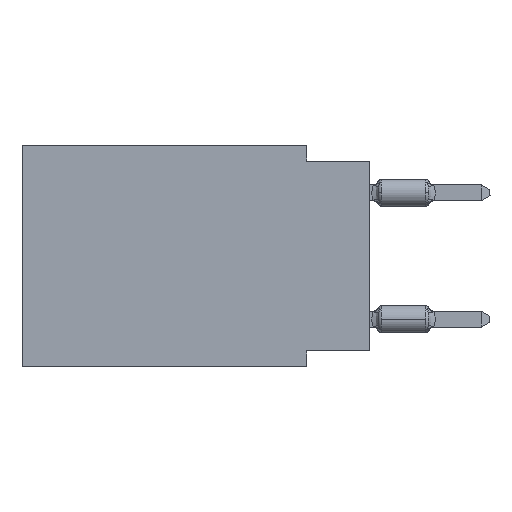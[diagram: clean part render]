
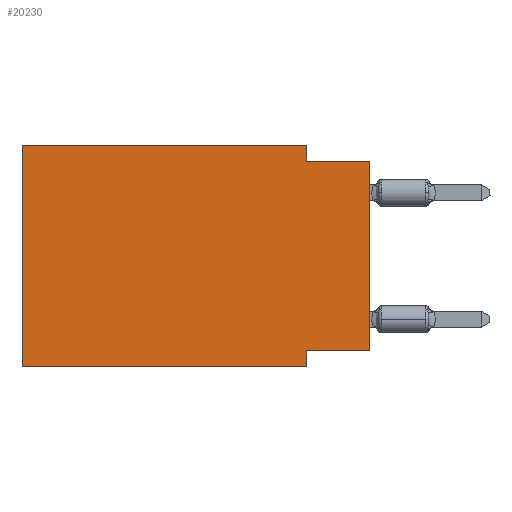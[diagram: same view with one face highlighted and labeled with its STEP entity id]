
A CAD part, left-side view. The second image highlights one B-rep face of the part: STEP entity #20230.
In plain terms, the highlighted planar face has unit normal (-1, 0, 0).
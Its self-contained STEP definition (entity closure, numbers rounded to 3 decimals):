
#2097 = ORIENTED_EDGE ( 'NONE', *, *, #26305, .F. ) ;
#3138 = DIRECTION ( 'NONE',  ( 0., 0., -1. ) ) ;
#5677 = DIRECTION ( 'NONE',  ( 0., 0., 1. ) ) ;
#6552 = VECTOR ( 'NONE', #24361, 1000. ) ;
#7790 = VERTEX_POINT ( 'NONE', #34208 ) ;
#7819 = VERTEX_POINT ( 'NONE', #51799 ) ;
#8036 = DIRECTION ( 'NONE',  ( 0., 0., 1. ) ) ;
#8139 = PLANE ( 'NONE',  #22504 ) ;
#8449 = EDGE_CURVE ( 'NONE', #12016, #8752, #50007, .T. ) ;
#8752 = VERTEX_POINT ( 'NONE', #41822 ) ;
#9020 = CARTESIAN_POINT ( 'NONE',  ( 0., 0., -8.255 ) ) ;
#9498 = VECTOR ( 'NONE', #8036, 1000. ) ;
#11505 = DIRECTION ( 'NONE',  ( 1., 0., 0. ) ) ;
#11742 = DIRECTION ( 'NONE',  ( 0., -1., 0. ) ) ;
#11849 = DIRECTION ( 'NONE',  ( 0., 0., -1. ) ) ;
#12016 = VERTEX_POINT ( 'NONE', #45140 ) ;
#12911 = ORIENTED_EDGE ( 'NONE', *, *, #34334, .F. ) ;
#14203 = LINE ( 'NONE', #52180, #38190 ) ;
#15864 = DIRECTION ( 'NONE',  ( 0., -1., 0. ) ) ;
#16439 = LINE ( 'NONE', #50491, #9498 ) ;
#16615 = LINE ( 'NONE', #45645, #28843 ) ;
#16933 = VECTOR ( 'NONE', #5677, 1000. ) ;
#17083 = EDGE_CURVE ( 'NONE', #34584, #38993, #52206, .T. ) ;
#18524 = ORIENTED_EDGE ( 'NONE', *, *, #28171, .F. ) ;
#19022 = CARTESIAN_POINT ( 'NONE',  ( 0., 2.54, 0. ) ) ;
#20230 = ADVANCED_FACE ( 'NONE', ( #20989 ), #8139, .F. ) ;
#20989 = FACE_OUTER_BOUND ( 'NONE', #37066, .T. ) ;
#21050 = EDGE_CURVE ( 'NONE', #7819, #38993, #36516, .T. ) ;
#22504 = AXIS2_PLACEMENT_3D ( 'NONE', #55076, #11505, #3138 ) ;
#23201 = LINE ( 'NONE', #19022, #30784 ) ;
#24361 = DIRECTION ( 'NONE',  ( 0., -1., 0. ) ) ;
#25776 = ORIENTED_EDGE ( 'NONE', *, *, #17083, .T. ) ;
#25944 = CARTESIAN_POINT ( 'NONE',  ( 0., 0., 0. ) ) ;
#26305 = EDGE_CURVE ( 'NONE', #12016, #47183, #16439, .T. ) ;
#26864 = VERTEX_POINT ( 'NONE', #39306 ) ;
#27538 = ORIENTED_EDGE ( 'NONE', *, *, #36419, .F. ) ;
#27926 = VECTOR ( 'NONE', #15864, 1000. ) ;
#28171 = EDGE_CURVE ( 'NONE', #34584, #26864, #14203, .T. ) ;
#28843 = VECTOR ( 'NONE', #11849, 1000. ) ;
#28976 = CARTESIAN_POINT ( 'NONE',  ( 0., 0., -0.635 ) ) ;
#30784 = VECTOR ( 'NONE', #36046, 1000. ) ;
#32564 = CARTESIAN_POINT ( 'NONE',  ( 0., 0., -0.635 ) ) ;
#34208 = CARTESIAN_POINT ( 'NONE',  ( 0., 2.54, 0. ) ) ;
#34230 = VECTOR ( 'NONE', #11742, 1000. ) ;
#34334 = EDGE_CURVE ( 'NONE', #26864, #8752, #16615, .T. ) ;
#34584 = VERTEX_POINT ( 'NONE', #9020 ) ;
#36046 = DIRECTION ( 'NONE',  ( 0., 0., -1. ) ) ;
#36419 = EDGE_CURVE ( 'NONE', #7790, #7819, #23201, .T. ) ;
#36516 = LINE ( 'NONE', #28976, #27926 ) ;
#37066 = EDGE_LOOP ( 'NONE', ( #25776, #39936, #27538, #48521, #2097, #49843, #12911, #18524 ) ) ;
#38190 = VECTOR ( 'NONE', #42952, 1000. ) ;
#38411 = CARTESIAN_POINT ( 'NONE',  ( 0., 13.97, 0. ) ) ;
#38993 = VERTEX_POINT ( 'NONE', #32564 ) ;
#39306 = CARTESIAN_POINT ( 'NONE',  ( 0., 2.54, -8.255 ) ) ;
#39936 = ORIENTED_EDGE ( 'NONE', *, *, #21050, .F. ) ;
#41822 = CARTESIAN_POINT ( 'NONE',  ( 0., 2.54, -8.89 ) ) ;
#42952 = DIRECTION ( 'NONE',  ( 0., 1., 0. ) ) ;
#45058 = LINE ( 'NONE', #49230, #6552 ) ;
#45140 = CARTESIAN_POINT ( 'NONE',  ( 0., 13.97, -8.89 ) ) ;
#45556 = CARTESIAN_POINT ( 'NONE',  ( 0., 13.97, -8.89 ) ) ;
#45645 = CARTESIAN_POINT ( 'NONE',  ( 0., 2.54, -8.89 ) ) ;
#47183 = VERTEX_POINT ( 'NONE', #38411 ) ;
#48521 = ORIENTED_EDGE ( 'NONE', *, *, #54580, .F. ) ;
#49230 = CARTESIAN_POINT ( 'NONE',  ( 0., 13.97, 0. ) ) ;
#49843 = ORIENTED_EDGE ( 'NONE', *, *, #8449, .T. ) ;
#50007 = LINE ( 'NONE', #45556, #34230 ) ;
#50491 = CARTESIAN_POINT ( 'NONE',  ( 0., 13.97, 0. ) ) ;
#51799 = CARTESIAN_POINT ( 'NONE',  ( 0., 2.54, -0.635 ) ) ;
#52180 = CARTESIAN_POINT ( 'NONE',  ( 0., 0., -8.255 ) ) ;
#52206 = LINE ( 'NONE', #25944, #16933 ) ;
#54580 = EDGE_CURVE ( 'NONE', #47183, #7790, #45058, .T. ) ;
#55076 = CARTESIAN_POINT ( 'NONE',  ( 0., 13.97, 0. ) ) ;
